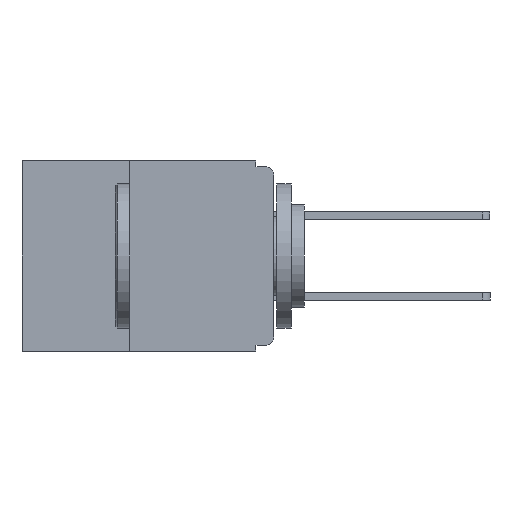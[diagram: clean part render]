
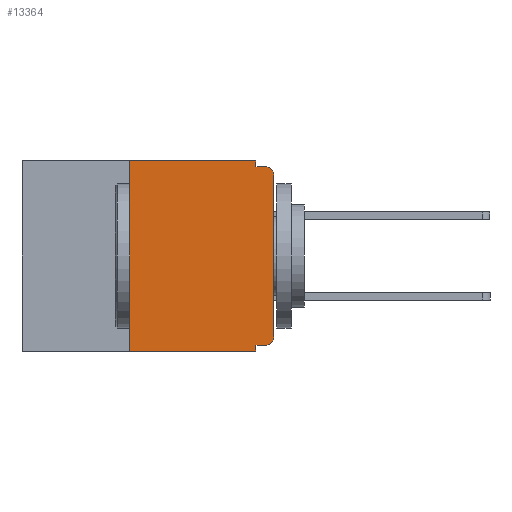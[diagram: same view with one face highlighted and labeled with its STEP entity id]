
A CAD part, left-side view. The second image highlights one B-rep face of the part: STEP entity #13364.
In plain terms, the highlighted planar face has unit normal (-1, 0, 0).
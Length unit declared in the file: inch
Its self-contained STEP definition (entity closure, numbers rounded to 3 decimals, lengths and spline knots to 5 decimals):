
#21 = VECTOR ( 'NONE', #21044, 39.37008 ) ;
#189 = VERTEX_POINT ( 'NONE', #17037 ) ;
#985 = CARTESIAN_POINT ( 'NONE',  ( 0., 0., -0.01 ) ) ;
#1111 = AXIS2_PLACEMENT_3D ( 'NONE', #5610, #13096, #1807 ) ;
#1306 = CARTESIAN_POINT ( 'NONE',  ( 0., 0.25, 0. ) ) ;
#1522 = ORIENTED_EDGE ( 'NONE', *, *, #23767, .F. ) ;
#1733 = DIRECTION ( 'NONE',  ( -1., 0., 0. ) ) ;
#1807 = DIRECTION ( 'NONE',  ( 0., 0., -1. ) ) ;
#1969 = EDGE_LOOP ( 'NONE', ( #23687, #9153, #21109, #6674, #1522, #2389, #3080, #17010, #23151, #3670 ) ) ;
#2025 = CARTESIAN_POINT ( 'NONE',  ( 0., 0.031, 0. ) ) ;
#2389 = ORIENTED_EDGE ( 'NONE', *, *, #23492, .F. ) ;
#2707 = CARTESIAN_POINT ( 'NONE',  ( 0., 0.015, -0.32 ) ) ;
#2750 = DIRECTION ( 'NONE',  ( -1., 0., 0. ) ) ;
#2876 = LINE ( 'NONE', #3647, #8001 ) ;
#3080 = ORIENTED_EDGE ( 'NONE', *, *, #22287, .T. ) ;
#3647 = CARTESIAN_POINT ( 'NONE',  ( 0., 0.031, -0.33 ) ) ;
#3670 = ORIENTED_EDGE ( 'NONE', *, *, #9658, .T. ) ;
#4706 = EDGE_CURVE ( 'NONE', #15206, #17694, #10185, .T. ) ;
#4856 = CIRCLE ( 'NONE', #19008, 0.015 ) ;
#5033 = VERTEX_POINT ( 'NONE', #2707 ) ;
#5118 = VECTOR ( 'NONE', #12300, 39.37008 ) ;
#5610 = CARTESIAN_POINT ( 'NONE',  ( 0., 0.437, 0. ) ) ;
#6065 = CARTESIAN_POINT ( 'NONE',  ( 0., 0.015, -0.01 ) ) ;
#6529 = CIRCLE ( 'NONE', #13965, 0.015 ) ;
#6674 = ORIENTED_EDGE ( 'NONE', *, *, #4706, .F. ) ;
#7439 = DIRECTION ( 'NONE',  ( 0., 0., 1. ) ) ;
#7618 = CARTESIAN_POINT ( 'NONE',  ( 0., 0.437, 0. ) ) ;
#7997 = VERTEX_POINT ( 'NONE', #12880 ) ;
#8001 = VECTOR ( 'NONE', #16665, 39.37008 ) ;
#8422 = CARTESIAN_POINT ( 'NONE',  ( 0., 0.437, -0.33 ) ) ;
#8706 = VECTOR ( 'NONE', #9482, 39.37008 ) ;
#9153 = ORIENTED_EDGE ( 'NONE', *, *, #13337, .T. ) ;
#9168 = CARTESIAN_POINT ( 'NONE',  ( 0., 0.031, 0. ) ) ;
#9246 = VECTOR ( 'NONE', #14856, 39.37008 ) ;
#9267 = DIRECTION ( 'NONE',  ( 0., 0., -1. ) ) ;
#9482 = DIRECTION ( 'NONE',  ( 0., -1., 0. ) ) ;
#9658 = EDGE_CURVE ( 'NONE', #5033, #19871, #6529, .T. ) ;
#10185 = LINE ( 'NONE', #9168, #23391 ) ;
#10415 = EDGE_CURVE ( 'NONE', #19871, #14341, #19648, .T. ) ;
#11002 = CARTESIAN_POINT ( 'NONE',  ( 0., 0., -0.305 ) ) ;
#12300 = DIRECTION ( 'NONE',  ( 0., 0., 1. ) ) ;
#12880 = CARTESIAN_POINT ( 'NONE',  ( 0., 0.031, -0.33 ) ) ;
#13018 = CARTESIAN_POINT ( 'NONE',  ( 0., 0.015, -0.025 ) ) ;
#13096 = DIRECTION ( 'NONE',  ( 1., 0., 0. ) ) ;
#13337 = EDGE_CURVE ( 'NONE', #14341, #20699, #4856, .T. ) ;
#13364 = ADVANCED_FACE ( 'NONE', ( #18436 ), #23784, .F. ) ;
#13965 = AXIS2_PLACEMENT_3D ( 'NONE', #13972, #2750, #15797 ) ;
#13972 = CARTESIAN_POINT ( 'NONE',  ( 0., 0.015, -0.305 ) ) ;
#14276 = CARTESIAN_POINT ( 'NONE',  ( 0., 0., -0.025 ) ) ;
#14341 = VERTEX_POINT ( 'NONE', #14276 ) ;
#14832 = DIRECTION ( 'NONE',  ( 0., 0., -1. ) ) ;
#14856 = DIRECTION ( 'NONE',  ( 0., 1., 0. ) ) ;
#14989 = LINE ( 'NONE', #21228, #5118 ) ;
#15206 = VERTEX_POINT ( 'NONE', #2025 ) ;
#15767 = EDGE_CURVE ( 'NONE', #5033, #22592, #18357, .T. ) ;
#15797 = DIRECTION ( 'NONE',  ( 0., 0., -1. ) ) ;
#15983 = DIRECTION ( 'NONE',  ( 0., -1., 0. ) ) ;
#16022 = VECTOR ( 'NONE', #7439, 39.37008 ) ;
#16665 = DIRECTION ( 'NONE',  ( 0., 0., -1. ) ) ;
#16955 = VERTEX_POINT ( 'NONE', #1306 ) ;
#17010 = ORIENTED_EDGE ( 'NONE', *, *, #19952, .F. ) ;
#17037 = CARTESIAN_POINT ( 'NONE',  ( 0., 0.25, -0.33 ) ) ;
#17694 = VERTEX_POINT ( 'NONE', #21836 ) ;
#18171 = LINE ( 'NONE', #8422, #21 ) ;
#18357 = LINE ( 'NONE', #20259, #9246 ) ;
#18383 = LINE ( 'NONE', #7618, #8706 ) ;
#18436 = FACE_OUTER_BOUND ( 'NONE', #1969, .T. ) ;
#18973 = VECTOR ( 'NONE', #15983, 39.37008 ) ;
#19008 = AXIS2_PLACEMENT_3D ( 'NONE', #13018, #1733, #14832 ) ;
#19532 = LINE ( 'NONE', #985, #18973 ) ;
#19648 = LINE ( 'NONE', #20147, #16022 ) ;
#19871 = VERTEX_POINT ( 'NONE', #11002 ) ;
#19952 = EDGE_CURVE ( 'NONE', #22592, #7997, #2876, .T. ) ;
#20147 = CARTESIAN_POINT ( 'NONE',  ( 0., 0., 0. ) ) ;
#20259 = CARTESIAN_POINT ( 'NONE',  ( 0., 0., -0.32 ) ) ;
#20699 = VERTEX_POINT ( 'NONE', #6065 ) ;
#21044 = DIRECTION ( 'NONE',  ( 0., -1., 0. ) ) ;
#21109 = ORIENTED_EDGE ( 'NONE', *, *, #22914, .F. ) ;
#21228 = CARTESIAN_POINT ( 'NONE',  ( 0., 0.25, -0.33 ) ) ;
#21836 = CARTESIAN_POINT ( 'NONE',  ( 0., 0.031, -0.01 ) ) ;
#22125 = CARTESIAN_POINT ( 'NONE',  ( 0., 0.031, -0.32 ) ) ;
#22287 = EDGE_CURVE ( 'NONE', #189, #7997, #18171, .T. ) ;
#22592 = VERTEX_POINT ( 'NONE', #22125 ) ;
#22914 = EDGE_CURVE ( 'NONE', #17694, #20699, #19532, .T. ) ;
#23151 = ORIENTED_EDGE ( 'NONE', *, *, #15767, .F. ) ;
#23391 = VECTOR ( 'NONE', #9267, 39.37008 ) ;
#23492 = EDGE_CURVE ( 'NONE', #189, #16955, #14989, .T. ) ;
#23687 = ORIENTED_EDGE ( 'NONE', *, *, #10415, .T. ) ;
#23767 = EDGE_CURVE ( 'NONE', #16955, #15206, #18383, .T. ) ;
#23784 = PLANE ( 'NONE',  #1111 ) ;
